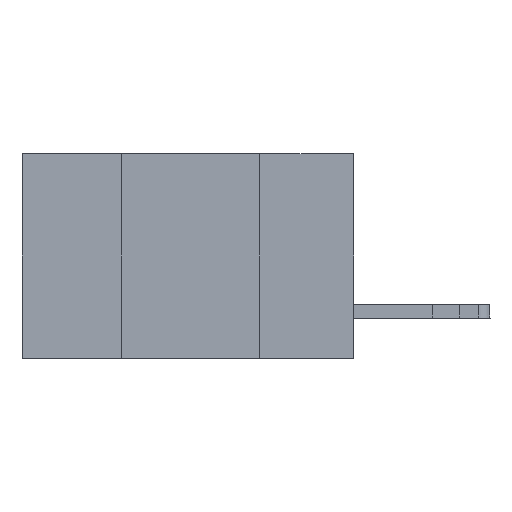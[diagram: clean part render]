
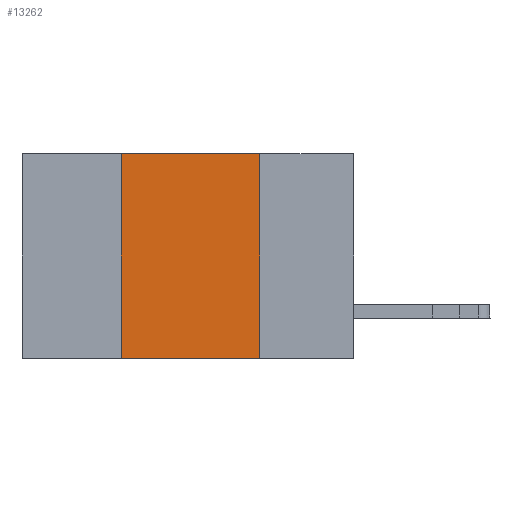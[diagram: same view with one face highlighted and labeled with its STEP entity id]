
A CAD part, left-side view. The second image highlights one B-rep face of the part: STEP entity #13262.
In plain terms, the highlighted planar face has unit normal (-1, 0, 0).
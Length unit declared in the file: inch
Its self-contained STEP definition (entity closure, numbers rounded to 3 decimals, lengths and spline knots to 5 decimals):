
#31 = CARTESIAN_POINT ( 'NONE',  ( 0., 0.42, 0. ) ) ;
#1067 = ORIENTED_EDGE ( 'NONE', *, *, #25300, .F. ) ;
#1704 = VERTEX_POINT ( 'NONE', #31 ) ;
#1710 = CARTESIAN_POINT ( 'NONE',  ( 0., 0.42, 0. ) ) ;
#1881 = CARTESIAN_POINT ( 'NONE',  ( 0., 0.17, -0.37 ) ) ;
#2006 = CARTESIAN_POINT ( 'NONE',  ( 0., 0.6, 0. ) ) ;
#3040 = ORIENTED_EDGE ( 'NONE', *, *, #20800, .F. ) ;
#6717 = VERTEX_POINT ( 'NONE', #28493 ) ;
#7336 = LINE ( 'NONE', #1710, #26642 ) ;
#11455 = DIRECTION ( 'NONE',  ( 0., -1., 0. ) ) ;
#13262 = ADVANCED_FACE ( 'NONE', ( #35752 ), #26854, .F. ) ;
#15241 = DIRECTION ( 'NONE',  ( 1., 0., 0. ) ) ;
#15615 = EDGE_LOOP ( 'NONE', ( #1067, #3040, #36543, #18048 ) ) ;
#17437 = VECTOR ( 'NONE', #37950, 39.37008 ) ;
#17940 = CARTESIAN_POINT ( 'NONE',  ( 0., 0.6, 0. ) ) ;
#18048 = ORIENTED_EDGE ( 'NONE', *, *, #33326, .T. ) ;
#20800 = EDGE_CURVE ( 'NONE', #1704, #6717, #28536, .T. ) ;
#23045 = LINE ( 'NONE', #37567, #17437 ) ;
#23153 = AXIS2_PLACEMENT_3D ( 'NONE', #17940, #15241, #24521 ) ;
#24085 = EDGE_CURVE ( 'NONE', #33981, #1704, #7336, .T. ) ;
#24318 = VECTOR ( 'NONE', #34800, 39.37008 ) ;
#24521 = DIRECTION ( 'NONE',  ( 0., 0., -1. ) ) ;
#25157 = VERTEX_POINT ( 'NONE', #1881 ) ;
#25300 = EDGE_CURVE ( 'NONE', #6717, #25157, #23045, .T. ) ;
#26642 = VECTOR ( 'NONE', #31529, 39.37008 ) ;
#26854 = PLANE ( 'NONE',  #23153 ) ;
#28493 = CARTESIAN_POINT ( 'NONE',  ( 0., 0.17, 0. ) ) ;
#28536 = LINE ( 'NONE', #2006, #34000 ) ;
#28791 = LINE ( 'NONE', #31511, #24318 ) ;
#31511 = CARTESIAN_POINT ( 'NONE',  ( 0., 0.6, -0.37 ) ) ;
#31529 = DIRECTION ( 'NONE',  ( 0., 0., 1. ) ) ;
#32836 = CARTESIAN_POINT ( 'NONE',  ( 0., 0.42, -0.37 ) ) ;
#33326 = EDGE_CURVE ( 'NONE', #33981, #25157, #28791, .T. ) ;
#33981 = VERTEX_POINT ( 'NONE', #32836 ) ;
#34000 = VECTOR ( 'NONE', #11455, 39.37008 ) ;
#34800 = DIRECTION ( 'NONE',  ( 0., -1., 0. ) ) ;
#35752 = FACE_OUTER_BOUND ( 'NONE', #15615, .T. ) ;
#36543 = ORIENTED_EDGE ( 'NONE', *, *, #24085, .F. ) ;
#37567 = CARTESIAN_POINT ( 'NONE',  ( 0., 0.17, 0. ) ) ;
#37950 = DIRECTION ( 'NONE',  ( 0., 0., -1. ) ) ;
